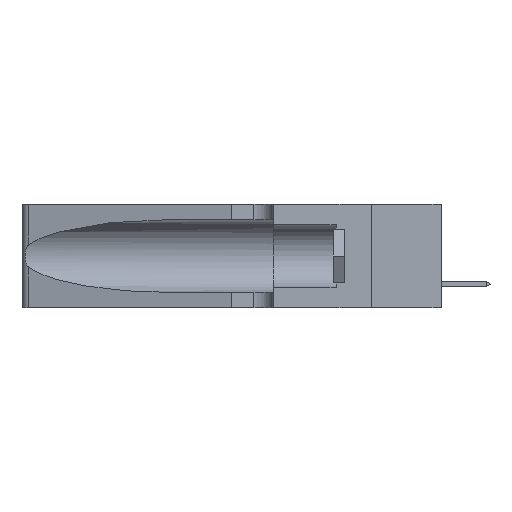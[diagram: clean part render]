
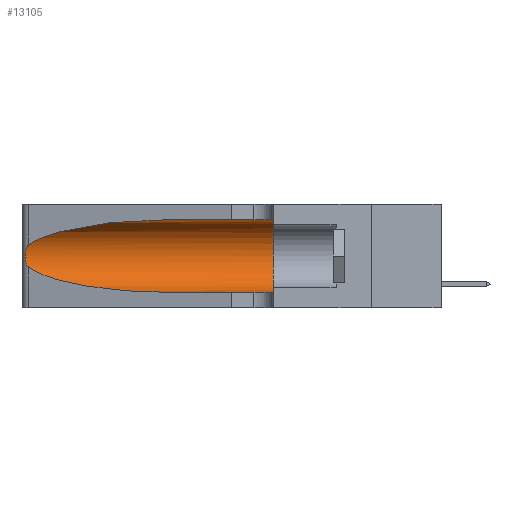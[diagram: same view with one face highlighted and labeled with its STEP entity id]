
A CAD part, left-side view. The second image highlights one B-rep face of the part: STEP entity #13105.
In plain terms, the highlighted cylindrical face has radius 3.308 mm (diameter 6.617 mm), a partial arc.
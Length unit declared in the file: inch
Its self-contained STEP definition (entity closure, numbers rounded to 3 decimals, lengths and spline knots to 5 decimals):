
#682 = CARTESIAN_POINT ( 'NONE',  ( 0.25487, 1.22718, 0.22369 ) ) ;
#1576 = VERTEX_POINT ( 'NONE', #18479 ) ;
#1589 = EDGE_CURVE ( 'NONE', #1576, #15203, #16454, .T. ) ;
#1708 = CARTESIAN_POINT ( 'NONE',  ( 0.1305, 0.72297, 0.31525 ) ) ;
#1786 = EDGE_CURVE ( 'NONE', #15203, #14311, #11276, .T. ) ;
#1818 = DIRECTION ( 'NONE',  ( 0., -1., 0. ) ) ;
#1893 = LINE ( 'NONE', #19243, #19101 ) ;
#2069 = AXIS2_PLACEMENT_3D ( 'NONE', #16101, #15969, #19543 ) ;
#2740 = CARTESIAN_POINT ( 'NONE',  ( 0.25487, 1.22718, 0.22369 ) ) ;
#2825 = CIRCLE ( 'NONE', #2069, 0.13025 ) ;
#3404 = AXIS2_PLACEMENT_3D ( 'NONE', #10105, #1818, #15092 ) ;
#3919 = CARTESIAN_POINT ( 'NONE',  ( 0.25639, 1.23184, 0.21858 ) ) ;
#4910 = LINE ( 'NONE', #16015, #11943 ) ;
#5361 = CARTESIAN_POINT ( 'NONE',  ( 0.25487, 1.22718, 0.14631 ) ) ;
#5601 = CARTESIAN_POINT ( 'NONE',  ( 0.25854, 1.2359, 0.20912 ) ) ;
#5679 = CARTESIAN_POINT ( 'NONE',  ( 0.25856, 1.23593, 0.16098 ) ) ;
#5778 = DIRECTION ( 'NONE',  ( 0., -1., 0. ) ) ;
#6029 = CARTESIAN_POINT ( 'NONE',  ( 0.25639, 1.23186, 0.15144 ) ) ;
#6144 = CARTESIAN_POINT ( 'NONE',  ( 0.25487, 1.22718, 0.14631 ) ) ;
#6753 =( BOUNDED_CURVE ( )  B_SPLINE_CURVE ( 3, ( #16156, #11154, #17767, #2740 ),
 .UNSPECIFIED., .F., .F. ) 
 B_SPLINE_CURVE_WITH_KNOTS ( ( 4, 4 ),
 ( 1.5708, 2.84003 ),
 .UNSPECIFIED. ) 
 CURVE ( )  GEOMETRIC_REPRESENTATION_ITEM ( )  RATIONAL_B_SPLINE_CURVE ( ( 1., 0.87, 0.87, 1. ) ) 
 REPRESENTATION_ITEM ( '' )  );
#6814 = ORIENTED_EDGE ( 'NONE', *, *, #16729, .T. ) ;
#6820 = EDGE_LOOP ( 'NONE', ( #6814, #10505, #9094, #14712, #12708, #12523 ) ) ;
#7269 = CARTESIAN_POINT ( 'NONE',  ( 0.26018, 1.23835, 0.19895 ) ) ;
#7622 = VERTEX_POINT ( 'NONE', #18497 ) ;
#7703 = CARTESIAN_POINT ( 'NONE',  ( 0.25555, 1.22993, 0.14849 ) ) ;
#8155 = CARTESIAN_POINT ( 'NONE',  ( 0.18966, 0.96281, 0.05475 ) ) ;
#8741 = VERTEX_POINT ( 'NONE', #1708 ) ;
#8957 = CARTESIAN_POINT ( 'NONE',  ( 0.26075, 1.23896, 0.178 ) ) ;
#9094 = ORIENTED_EDGE ( 'NONE', *, *, #1786, .T. ) ;
#10105 = CARTESIAN_POINT ( 'NONE',  ( 0.1305, 1.61858, 0.185 ) ) ;
#10505 = ORIENTED_EDGE ( 'NONE', *, *, #1589, .T. ) ;
#10834 = CARTESIAN_POINT ( 'NONE',  ( 0.25789, 1.23486, 0.15765 ) ) ;
#11154 = CARTESIAN_POINT ( 'NONE',  ( 0.18966, 0.96281, 0.31525 ) ) ;
#11222 = DIRECTION ( 'NONE',  ( 0., -1., 0. ) ) ;
#11276 =( BOUNDED_CURVE ( )  B_SPLINE_CURVE ( 3, ( #6144, #12814, #8155, #19655 ),
 .UNSPECIFIED., .F., .F. ) 
 B_SPLINE_CURVE_WITH_KNOTS ( ( 4, 4 ),
 ( 3.44316, 4.71239 ),
 .UNSPECIFIED. ) 
 CURVE ( )  GEOMETRIC_REPRESENTATION_ITEM ( )  RATIONAL_B_SPLINE_CURVE ( ( 1., 0.87, 0.87, 1. ) ) 
 REPRESENTATION_ITEM ( '' )  );
#11350 = EDGE_CURVE ( 'NONE', #8741, #18117, #1893, .T. ) ;
#11943 = VECTOR ( 'NONE', #11222, 39.37008 ) ;
#11983 = CARTESIAN_POINT ( 'NONE',  ( 0.1305, 0.35, 0.31525 ) ) ;
#12508 = FACE_OUTER_BOUND ( 'NONE', #6820, .T. ) ;
#12523 = ORIENTED_EDGE ( 'NONE', *, *, #11350, .F. ) ;
#12708 = ORIENTED_EDGE ( 'NONE', *, *, #17108, .F. ) ;
#12814 = CARTESIAN_POINT ( 'NONE',  ( 0.2373, 1.15595, 0.08982 ) ) ;
#13105 = ADVANCED_FACE ( 'NONE', ( #12508 ), #17187, .F. ) ;
#13860 = CARTESIAN_POINT ( 'NONE',  ( 0.25555, 1.22994, 0.2215 ) ) ;
#14311 = VERTEX_POINT ( 'NONE', #15950 ) ;
#14712 = ORIENTED_EDGE ( 'NONE', *, *, #16554, .T. ) ;
#15092 = DIRECTION ( 'NONE',  ( 0., 0., -1. ) ) ;
#15203 = VERTEX_POINT ( 'NONE', #5361 ) ;
#15606 = CARTESIAN_POINT ( 'NONE',  ( 0.25787, 1.23484, 0.2124 ) ) ;
#15950 = CARTESIAN_POINT ( 'NONE',  ( 0.1305, 0.72297, 0.05475 ) ) ;
#15969 = DIRECTION ( 'NONE',  ( 0., 1., 0. ) ) ;
#16015 = CARTESIAN_POINT ( 'NONE',  ( 0.1305, 1.61858, 0.05475 ) ) ;
#16034 = CARTESIAN_POINT ( 'NONE',  ( 0.25487, 1.22718, 0.14631 ) ) ;
#16101 = CARTESIAN_POINT ( 'NONE',  ( 0.1305, 0.35, 0.185 ) ) ;
#16156 = CARTESIAN_POINT ( 'NONE',  ( 0.1305, 0.72297, 0.31525 ) ) ;
#16454 = B_SPLINE_CURVE_WITH_KNOTS ( 'NONE', 3,
 ( #682, #13860, #3919, #15606, #5601, #7269, #18921, #8957, #20599, #5679, #10834, #6029, #7703, #16034 ),
 .UNSPECIFIED., .F., .F.,
 ( 4, 2, 2, 2, 2, 2, 4 ),
 ( 0., 0.00027, 0.00053, 0.00107, 0.0016, 0.00187, 0.00214 ),
 .UNSPECIFIED. ) ;
#16554 = EDGE_CURVE ( 'NONE', #14311, #7622, #4910, .T. ) ;
#16729 = EDGE_CURVE ( 'NONE', #8741, #1576, #6753, .T. ) ;
#17108 = EDGE_CURVE ( 'NONE', #18117, #7622, #2825, .T. ) ;
#17187 = CYLINDRICAL_SURFACE ( 'NONE', #3404, 0.13025 ) ;
#17767 = CARTESIAN_POINT ( 'NONE',  ( 0.2373, 1.15595, 0.28018 ) ) ;
#18117 = VERTEX_POINT ( 'NONE', #11983 ) ;
#18479 = CARTESIAN_POINT ( 'NONE',  ( 0.25487, 1.22718, 0.22369 ) ) ;
#18497 = CARTESIAN_POINT ( 'NONE',  ( 0.1305, 0.35, 0.05475 ) ) ;
#18921 = CARTESIAN_POINT ( 'NONE',  ( 0.26075, 1.23896, 0.19203 ) ) ;
#19101 = VECTOR ( 'NONE', #5778, 39.37008 ) ;
#19243 = CARTESIAN_POINT ( 'NONE',  ( 0.1305, 1.61858, 0.31525 ) ) ;
#19543 = DIRECTION ( 'NONE',  ( 0., 0., 1. ) ) ;
#19655 = CARTESIAN_POINT ( 'NONE',  ( 0.1305, 0.72297, 0.05475 ) ) ;
#20599 = CARTESIAN_POINT ( 'NONE',  ( 0.26017, 1.23833, 0.17102 ) ) ;
